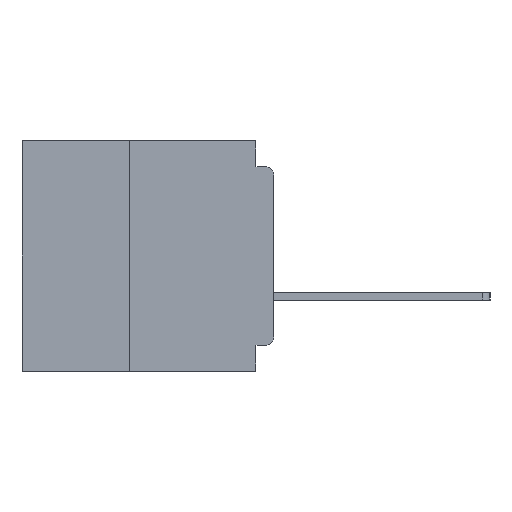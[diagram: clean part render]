
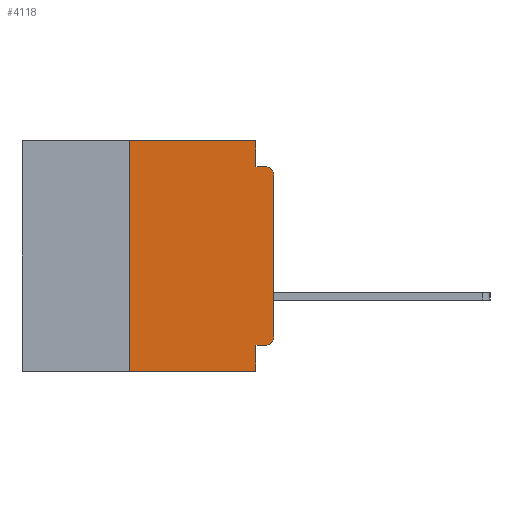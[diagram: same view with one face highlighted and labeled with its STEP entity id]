
A CAD part, left-side view. The second image highlights one B-rep face of the part: STEP entity #4118.
In plain terms, the highlighted planar face has unit normal (-1, 0, 0).
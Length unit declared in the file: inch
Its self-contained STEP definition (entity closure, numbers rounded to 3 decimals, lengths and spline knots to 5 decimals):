
#372 = VERTEX_POINT ( 'NONE', #14150 ) ;
#674 = EDGE_CURVE ( 'NONE', #33213, #22174, #33272, .T. ) ;
#1401 = LINE ( 'NONE', #22987, #27618 ) ;
#1744 = DIRECTION ( 'NONE',  ( 0., 0., 1. ) ) ;
#1976 = VERTEX_POINT ( 'NONE', #38549 ) ;
#2031 = ORIENTED_EDGE ( 'NONE', *, *, #25419, .T. ) ;
#2255 = CARTESIAN_POINT ( 'NONE',  ( 0., 0.031, 0. ) ) ;
#2289 = DIRECTION ( 'NONE',  ( 0., -1., 0. ) ) ;
#3626 = ORIENTED_EDGE ( 'NONE', *, *, #42939, .F. ) ;
#4118 = ADVANCED_FACE ( 'NONE', ( #17584 ), #40847, .F. ) ;
#4140 = ORIENTED_EDGE ( 'NONE', *, *, #24782, .F. ) ;
#5192 = EDGE_CURVE ( 'NONE', #1976, #41916, #43295, .T. ) ;
#5592 = AXIS2_PLACEMENT_3D ( 'NONE', #37055, #16439, #40503 ) ;
#5966 = LINE ( 'NONE', #39892, #22002 ) ;
#6370 = VERTEX_POINT ( 'NONE', #32908 ) ;
#6652 = CARTESIAN_POINT ( 'NONE',  ( 0., 0.437, 0. ) ) ;
#7923 = AXIS2_PLACEMENT_3D ( 'NONE', #6652, #44420, #23861 ) ;
#9179 = DIRECTION ( 'NONE',  ( 0., 0., -1. ) ) ;
#9388 = ORIENTED_EDGE ( 'NONE', *, *, #5192, .F. ) ;
#10152 = CIRCLE ( 'NONE', #5592, 0.015 ) ;
#10396 = VECTOR ( 'NONE', #9179, 39.37008 ) ;
#11127 = EDGE_CURVE ( 'NONE', #17934, #22174, #10152, .T. ) ;
#11320 = VERTEX_POINT ( 'NONE', #33784 ) ;
#11523 = CARTESIAN_POINT ( 'NONE',  ( 0., 0., -0.355 ) ) ;
#12585 = DIRECTION ( 'NONE',  ( 0., 0., 1. ) ) ;
#14033 = AXIS2_PLACEMENT_3D ( 'NONE', #14232, #38325, #17702 ) ;
#14150 = CARTESIAN_POINT ( 'NONE',  ( 0., 0.015, -0.355 ) ) ;
#14232 = CARTESIAN_POINT ( 'NONE',  ( 0., 0.015, -0.34 ) ) ;
#14858 = ORIENTED_EDGE ( 'NONE', *, *, #26328, .F. ) ;
#15319 = DIRECTION ( 'NONE',  ( 0., -1., 0. ) ) ;
#15449 = CARTESIAN_POINT ( 'NONE',  ( 0., 0.031, -0.4 ) ) ;
#15934 = CARTESIAN_POINT ( 'NONE',  ( 0., 0.031, -0.4 ) ) ;
#15936 = DIRECTION ( 'NONE',  ( 0., -1., 0. ) ) ;
#16439 = DIRECTION ( 'NONE',  ( -1., 0., 0. ) ) ;
#16534 = CARTESIAN_POINT ( 'NONE',  ( 0., 0., -0.045 ) ) ;
#17584 = FACE_OUTER_BOUND ( 'NONE', #32236, .T. ) ;
#17666 = VECTOR ( 'NONE', #15319, 39.37008 ) ;
#17702 = DIRECTION ( 'NONE',  ( 0., 0., -1. ) ) ;
#17934 = VERTEX_POINT ( 'NONE', #20897 ) ;
#18435 = DIRECTION ( 'NONE',  ( 0., 1., 0. ) ) ;
#18541 = ORIENTED_EDGE ( 'NONE', *, *, #26866, .T. ) ;
#19492 = LINE ( 'NONE', #2255, #10396 ) ;
#19853 = VERTEX_POINT ( 'NONE', #43811 ) ;
#20897 = CARTESIAN_POINT ( 'NONE',  ( 0., 0., -0.06 ) ) ;
#22002 = VECTOR ( 'NONE', #2289, 39.37008 ) ;
#22011 = CARTESIAN_POINT ( 'NONE',  ( 0., 0.25, -0.4 ) ) ;
#22174 = VERTEX_POINT ( 'NONE', #32945 ) ;
#22987 = CARTESIAN_POINT ( 'NONE',  ( 0., 0., 0. ) ) ;
#23065 = VECTOR ( 'NONE', #15936, 39.37008 ) ;
#23861 = DIRECTION ( 'NONE',  ( 0., 0., -1. ) ) ;
#24782 = EDGE_CURVE ( 'NONE', #372, #1976, #43167, .T. ) ;
#24895 = VECTOR ( 'NONE', #18435, 39.37008 ) ;
#25419 = EDGE_CURVE ( 'NONE', #372, #11320, #43630, .T. ) ;
#26328 = EDGE_CURVE ( 'NONE', #27843, #6370, #5966, .T. ) ;
#26822 = LINE ( 'NONE', #35936, #17666 ) ;
#26866 = EDGE_CURVE ( 'NONE', #19853, #41916, #26822, .T. ) ;
#27618 = VECTOR ( 'NONE', #12585, 39.37008 ) ;
#27843 = VERTEX_POINT ( 'NONE', #31497 ) ;
#28912 = CARTESIAN_POINT ( 'NONE',  ( 0., 0.031, -0.045 ) ) ;
#29780 = DIRECTION ( 'NONE',  ( 0., 0., -1. ) ) ;
#31237 = VECTOR ( 'NONE', #1744, 39.37008 ) ;
#31497 = CARTESIAN_POINT ( 'NONE',  ( 0., 0.25, 0. ) ) ;
#32236 = EDGE_LOOP ( 'NONE', ( #33176, #36726, #38058, #33022, #14858, #3626, #18541, #9388, #4140, #2031 ) ) ;
#32908 = CARTESIAN_POINT ( 'NONE',  ( 0., 0.031, 0. ) ) ;
#32945 = CARTESIAN_POINT ( 'NONE',  ( 0., 0.015, -0.045 ) ) ;
#33022 = ORIENTED_EDGE ( 'NONE', *, *, #41505, .F. ) ;
#33176 = ORIENTED_EDGE ( 'NONE', *, *, #41527, .T. ) ;
#33213 = VERTEX_POINT ( 'NONE', #28912 ) ;
#33272 = LINE ( 'NONE', #16534, #23065 ) ;
#33784 = CARTESIAN_POINT ( 'NONE',  ( 0., 0., -0.34 ) ) ;
#34156 = VECTOR ( 'NONE', #29780, 39.37008 ) ;
#35936 = CARTESIAN_POINT ( 'NONE',  ( 0., 0.437, -0.4 ) ) ;
#36726 = ORIENTED_EDGE ( 'NONE', *, *, #11127, .T. ) ;
#37055 = CARTESIAN_POINT ( 'NONE',  ( 0., 0.015, -0.06 ) ) ;
#38058 = ORIENTED_EDGE ( 'NONE', *, *, #674, .F. ) ;
#38325 = DIRECTION ( 'NONE',  ( -1., 0., 0. ) ) ;
#38549 = CARTESIAN_POINT ( 'NONE',  ( 0., 0.031, -0.355 ) ) ;
#39892 = CARTESIAN_POINT ( 'NONE',  ( 0., 0.437, 0. ) ) ;
#40370 = LINE ( 'NONE', #22011, #31237 ) ;
#40503 = DIRECTION ( 'NONE',  ( 0., 0., -1. ) ) ;
#40847 = PLANE ( 'NONE',  #7923 ) ;
#41505 = EDGE_CURVE ( 'NONE', #6370, #33213, #19492, .T. ) ;
#41527 = EDGE_CURVE ( 'NONE', #11320, #17934, #1401, .T. ) ;
#41916 = VERTEX_POINT ( 'NONE', #15449 ) ;
#42939 = EDGE_CURVE ( 'NONE', #19853, #27843, #40370, .T. ) ;
#43167 = LINE ( 'NONE', #11523, #24895 ) ;
#43295 = LINE ( 'NONE', #15934, #34156 ) ;
#43630 = CIRCLE ( 'NONE', #14033, 0.015 ) ;
#43811 = CARTESIAN_POINT ( 'NONE',  ( 0., 0.25, -0.4 ) ) ;
#44420 = DIRECTION ( 'NONE',  ( 1., 0., 0. ) ) ;
